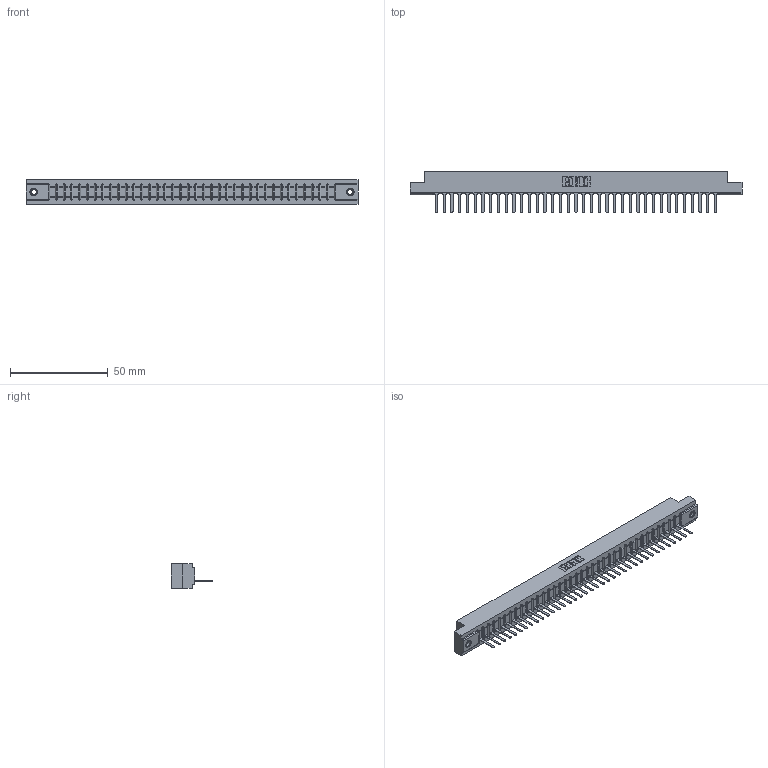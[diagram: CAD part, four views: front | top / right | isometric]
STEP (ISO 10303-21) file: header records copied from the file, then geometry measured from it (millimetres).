
FILE_DESCRIPTION (( 'STEP AP203' ), '1' );
FILE_NAME ('357-037-427-107.STEP', '2020-10-02T18:19:50', ( '' ), ( '' ), 'SwSTEP 2.0', 'SolidWorks 2020', '' );
FILE_SCHEMA (( 'CONFIG_CONTROL_DESIGN' ));
Length unit declared in the file: inch
Products named in the file (4): 307-290-001_527; 307 Part_.156 Dia Mounting Holes; 345-250-001_345-250-005-103; 357-037-427-107
Assembly tree (40 placements, depth 2):
  357-037-427-107
    307 Part_.156 Dia Mounting Holes
    307-290-001_527  x37
    345-250-001_345-250-005-103  x2
Bounding box: 169.62 x 21.11 x 12.7 mm (x, y, z)
Volume: 17590.6 mm3; surface area: 18725.1 mm2
Topology: 40 solids, 40 shells, 2288 faces, 6453 edges, 4142 vertices
Faces by surface type: plane 1471, cylinder 725, sphere 76, cone 12, torus 4
Entity records: 33489 total; most frequent: CARTESIAN_POINT 5619, ORIENTED_EDGE 5598, DIRECTION 5477, EDGE_CURVE 2799, LINE 2145, VECTOR 2145, VERTEX_POINT 1808, AXIS2_PLACEMENT_3D 1666
